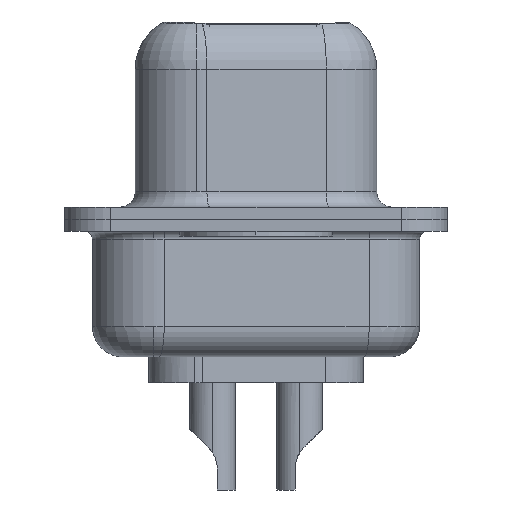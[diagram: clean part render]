
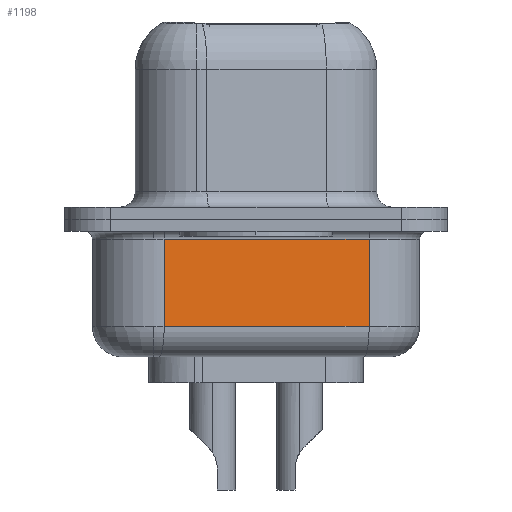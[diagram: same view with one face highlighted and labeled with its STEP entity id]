
A CAD part, left-side view. The second image highlights one B-rep face of the part: STEP entity #1198.
In plain terms, the highlighted planar face has unit normal (-0.985, -0.174, 0).
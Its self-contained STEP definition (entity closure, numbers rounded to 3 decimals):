
#150 = CARTESIAN_POINT ( 'NONE',  ( 4.062, -3.697, -3.5 ) ) ;
#552 = CARTESIAN_POINT ( 'NONE',  ( 2.88, 3.003, -3.5 ) ) ;
#772 = DIRECTION ( 'NONE',  ( 0., 0., 1. ) ) ;
#813 = DIRECTION ( 'NONE',  ( 0.174, -0.985, 0. ) ) ;
#1198 = ADVANCED_FACE ( 'NONE', ( #11518 ), #5086, .F. ) ;
#1390 = VERTEX_POINT ( 'NONE', #11857 ) ;
#1812 = CARTESIAN_POINT ( 'NONE',  ( 2.88, 3.003, -4.5 ) ) ;
#1910 = LINE ( 'NONE', #5177, #6381 ) ;
#2053 = EDGE_LOOP ( 'NONE', ( #12993, #10535, #9620, #8002 ) ) ;
#2855 = LINE ( 'NONE', #1812, #10930 ) ;
#2946 = CARTESIAN_POINT ( 'NONE',  ( 2.88, 3.003, -0.65 ) ) ;
#3639 = VERTEX_POINT ( 'NONE', #9668 ) ;
#3859 = LINE ( 'NONE', #2946, #7697 ) ;
#3885 = AXIS2_PLACEMENT_3D ( 'NONE', #10463, #13607, #8515 ) ;
#4331 = EDGE_CURVE ( 'NONE', #11852, #11802, #10439, .T. ) ;
#5086 = PLANE ( 'NONE',  #3885 ) ;
#5177 = CARTESIAN_POINT ( 'NONE',  ( 4.062, -3.697, -4.5 ) ) ;
#6381 = VECTOR ( 'NONE', #13558, 1000. ) ;
#7686 = EDGE_CURVE ( 'NONE', #11802, #3639, #1910, .T. ) ;
#7697 = VECTOR ( 'NONE', #11535, 1000. ) ;
#7743 = EDGE_CURVE ( 'NONE', #3639, #1390, #3859, .T. ) ;
#8002 = ORIENTED_EDGE ( 'NONE', *, *, #7743, .T. ) ;
#8425 = CARTESIAN_POINT ( 'NONE',  ( 2.88, 3.003, -3.5 ) ) ;
#8515 = DIRECTION ( 'NONE',  ( -0.174, 0.985, 0. ) ) ;
#8788 = VECTOR ( 'NONE', #813, 1000. ) ;
#9620 = ORIENTED_EDGE ( 'NONE', *, *, #7686, .T. ) ;
#9668 = CARTESIAN_POINT ( 'NONE',  ( 4.062, -3.697, -0.65 ) ) ;
#10439 = LINE ( 'NONE', #8425, #8788 ) ;
#10463 = CARTESIAN_POINT ( 'NONE',  ( 2.88, 3.003, -4.5 ) ) ;
#10535 = ORIENTED_EDGE ( 'NONE', *, *, #4331, .T. ) ;
#10930 = VECTOR ( 'NONE', #772, 1000. ) ;
#11518 = FACE_OUTER_BOUND ( 'NONE', #2053, .T. ) ;
#11535 = DIRECTION ( 'NONE',  ( -0.174, 0.985, 0. ) ) ;
#11698 = EDGE_CURVE ( 'NONE', #11852, #1390, #2855, .T. ) ;
#11802 = VERTEX_POINT ( 'NONE', #150 ) ;
#11852 = VERTEX_POINT ( 'NONE', #552 ) ;
#11857 = CARTESIAN_POINT ( 'NONE',  ( 2.88, 3.003, -0.65 ) ) ;
#12993 = ORIENTED_EDGE ( 'NONE', *, *, #11698, .F. ) ;
#13558 = DIRECTION ( 'NONE',  ( 0., 0., 1. ) ) ;
#13607 = DIRECTION ( 'NONE',  ( 0.985, 0.174, 0. ) ) ;
